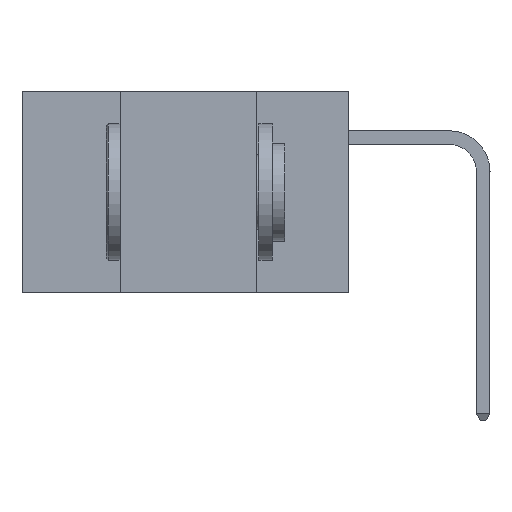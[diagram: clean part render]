
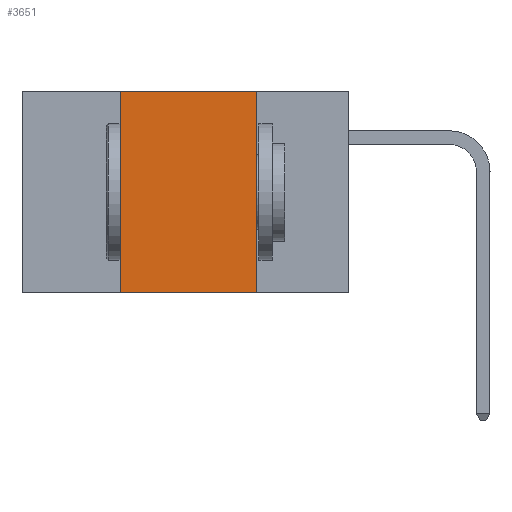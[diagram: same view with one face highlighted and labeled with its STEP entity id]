
A CAD part, left-side view. The second image highlights one B-rep face of the part: STEP entity #3651.
In plain terms, the highlighted planar face has unit normal (-1, 0, 0).
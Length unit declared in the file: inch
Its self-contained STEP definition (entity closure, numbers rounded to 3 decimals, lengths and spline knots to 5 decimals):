
#608 = EDGE_CURVE ( 'NONE', #19959, #3747, #8453, .T. ) ;
#1180 = CARTESIAN_POINT ( 'NONE',  ( 0., 0.17, -0.37 ) ) ;
#1699 = ORIENTED_EDGE ( 'NONE', *, *, #608, .T. ) ;
#1780 = EDGE_CURVE ( 'NONE', #19959, #4661, #9151, .T. ) ;
#2288 = CARTESIAN_POINT ( 'NONE',  ( 0., 0.42, -0.37 ) ) ;
#2787 = DIRECTION ( 'NONE',  ( 0., 0., -1. ) ) ;
#2838 = DIRECTION ( 'NONE',  ( 0., -1., 0. ) ) ;
#2842 = DIRECTION ( 'NONE',  ( 1., 0., 0. ) ) ;
#2975 = PLANE ( 'NONE',  #18607 ) ;
#3234 = CARTESIAN_POINT ( 'NONE',  ( 0., 0.6, 0. ) ) ;
#3651 = ADVANCED_FACE ( 'NONE', ( #3706 ), #2975, .F. ) ;
#3706 = FACE_OUTER_BOUND ( 'NONE', #15089, .T. ) ;
#3747 = VERTEX_POINT ( 'NONE', #1180 ) ;
#4051 = EDGE_CURVE ( 'NONE', #17685, #3747, #13701, .T. ) ;
#4442 = CARTESIAN_POINT ( 'NONE',  ( 0., 0.42, 0. ) ) ;
#4468 = DIRECTION ( 'NONE',  ( 0., 0., 1. ) ) ;
#4661 = VERTEX_POINT ( 'NONE', #18567 ) ;
#5117 = ORIENTED_EDGE ( 'NONE', *, *, #8908, .F. ) ;
#5925 = LINE ( 'NONE', #8256, #17497 ) ;
#8256 = CARTESIAN_POINT ( 'NONE',  ( 0., 0.6, 0. ) ) ;
#8453 = LINE ( 'NONE', #14482, #16252 ) ;
#8657 = VECTOR ( 'NONE', #4468, 39.37008 ) ;
#8908 = EDGE_CURVE ( 'NONE', #4661, #17685, #5925, .T. ) ;
#9151 = LINE ( 'NONE', #4442, #8657 ) ;
#9265 = CARTESIAN_POINT ( 'NONE',  ( 0., 0.17, 0. ) ) ;
#9847 = DIRECTION ( 'NONE',  ( 0., -1., 0. ) ) ;
#13194 = VECTOR ( 'NONE', #18292, 39.37008 ) ;
#13701 = LINE ( 'NONE', #18987, #13194 ) ;
#14058 = ORIENTED_EDGE ( 'NONE', *, *, #1780, .F. ) ;
#14482 = CARTESIAN_POINT ( 'NONE',  ( 0., 0.6, -0.37 ) ) ;
#15089 = EDGE_LOOP ( 'NONE', ( #20333, #5117, #14058, #1699 ) ) ;
#16252 = VECTOR ( 'NONE', #2838, 39.37008 ) ;
#17497 = VECTOR ( 'NONE', #9847, 39.37008 ) ;
#17685 = VERTEX_POINT ( 'NONE', #9265 ) ;
#18292 = DIRECTION ( 'NONE',  ( 0., 0., -1. ) ) ;
#18567 = CARTESIAN_POINT ( 'NONE',  ( 0., 0.42, 0. ) ) ;
#18607 = AXIS2_PLACEMENT_3D ( 'NONE', #3234, #2842, #2787 ) ;
#18987 = CARTESIAN_POINT ( 'NONE',  ( 0., 0.17, 0. ) ) ;
#19959 = VERTEX_POINT ( 'NONE', #2288 ) ;
#20333 = ORIENTED_EDGE ( 'NONE', *, *, #4051, .F. ) ;
